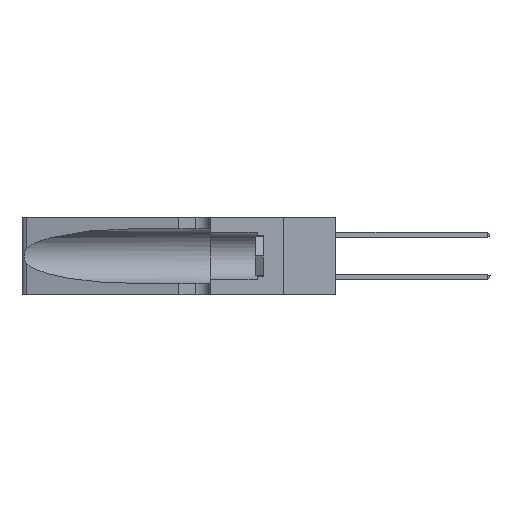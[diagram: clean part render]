
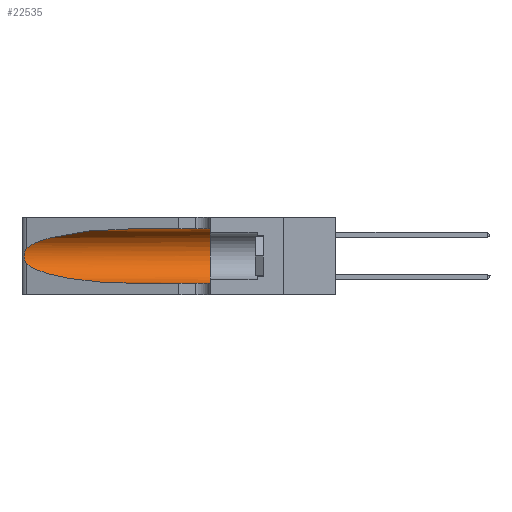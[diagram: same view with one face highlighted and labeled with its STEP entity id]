
A CAD part, left-side view. The second image highlights one B-rep face of the part: STEP entity #22535.
In plain terms, the highlighted cylindrical face has radius 3.308 mm (diameter 6.617 mm), a partial arc.
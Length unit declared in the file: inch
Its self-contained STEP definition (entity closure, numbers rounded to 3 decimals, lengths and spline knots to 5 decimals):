
#37 = ORIENTED_EDGE ( 'NONE', *, *, #28800, .T. ) ;
#1227 = DIRECTION ( 'NONE',  ( 0., 0., 1. ) ) ;
#1616 = CARTESIAN_POINT ( 'NONE',  ( 0.26075, 1.23896, 0.19203 ) ) ;
#3065 = CARTESIAN_POINT ( 'NONE',  ( 0.25487, 1.22718, 0.22369 ) ) ;
#3207 = VECTOR ( 'NONE', #26814, 39.37008 ) ;
#4339 = B_SPLINE_CURVE_WITH_KNOTS ( 'NONE', 3,
 ( #32997, #5074, #39997, #19116, #43518, #22631, #1616, #26113, #5220, #29603, #8793, #33145, #12297, #36642 ),
 .UNSPECIFIED., .F., .F.,
 ( 4, 2, 2, 2, 2, 2, 4 ),
 ( 0., 0.00027, 0.00053, 0.00107, 0.0016, 0.00187, 0.00214 ),
 .UNSPECIFIED. ) ;
#5074 = CARTESIAN_POINT ( 'NONE',  ( 0.25555, 1.22994, 0.2215 ) ) ;
#5168 = LINE ( 'NONE', #7777, #41179 ) ;
#5220 = CARTESIAN_POINT ( 'NONE',  ( 0.26017, 1.23833, 0.17102 ) ) ;
#5455 = LINE ( 'NONE', #9481, #3207 ) ;
#5785 = EDGE_CURVE ( 'NONE', #18991, #15738, #33452, .T. ) ;
#7057 = CARTESIAN_POINT ( 'NONE',  ( 0.18966, 0.96281, 0.05475 ) ) ;
#7777 = CARTESIAN_POINT ( 'NONE',  ( 0.1305, 1.61858, 0.05475 ) ) ;
#8030 = VERTEX_POINT ( 'NONE', #14000 ) ;
#8793 = CARTESIAN_POINT ( 'NONE',  ( 0.25789, 1.23486, 0.15765 ) ) ;
#9481 = CARTESIAN_POINT ( 'NONE',  ( 0.1305, 1.61858, 0.31525 ) ) ;
#12297 = CARTESIAN_POINT ( 'NONE',  ( 0.25555, 1.22993, 0.14849 ) ) ;
#14000 = CARTESIAN_POINT ( 'NONE',  ( 0.25487, 1.22718, 0.14631 ) ) ;
#15154 = AXIS2_PLACEMENT_3D ( 'NONE', #42741, #25344, #28840 ) ;
#15531 = ORIENTED_EDGE ( 'NONE', *, *, #22276, .T. ) ;
#15738 = VERTEX_POINT ( 'NONE', #21286 ) ;
#16546 = VERTEX_POINT ( 'NONE', #43029 ) ;
#17122 = EDGE_CURVE ( 'NONE', #23274, #15738, #5168, .T. ) ;
#18991 = VERTEX_POINT ( 'NONE', #23739 ) ;
#19116 = CARTESIAN_POINT ( 'NONE',  ( 0.25787, 1.23484, 0.2124 ) ) ;
#19890 = ORIENTED_EDGE ( 'NONE', *, *, #17122, .T. ) ;
#21286 = CARTESIAN_POINT ( 'NONE',  ( 0.1305, 0.35, 0.05475 ) ) ;
#21406 = VERTEX_POINT ( 'NONE', #36669 ) ;
#22077 = ORIENTED_EDGE ( 'NONE', *, *, #29671, .F. ) ;
#22264 = DIRECTION ( 'NONE',  ( 0., 1., 0. ) ) ;
#22276 = EDGE_CURVE ( 'NONE', #21406, #16546, #28641, .T. ) ;
#22535 = ADVANCED_FACE ( 'NONE', ( #31312 ), #23187, .F. ) ;
#22631 = CARTESIAN_POINT ( 'NONE',  ( 0.26018, 1.23835, 0.19895 ) ) ;
#23050 = CARTESIAN_POINT ( 'NONE',  ( 0.1305, 0.72297, 0.05475 ) ) ;
#23187 = CYLINDRICAL_SURFACE ( 'NONE', #15154, 0.13025 ) ;
#23274 = VERTEX_POINT ( 'NONE', #23050 ) ;
#23739 = CARTESIAN_POINT ( 'NONE',  ( 0.1305, 0.35, 0.31525 ) ) ;
#24008 = CARTESIAN_POINT ( 'NONE',  ( 0.2373, 1.15595, 0.28018 ) ) ;
#25263 = DIRECTION ( 'NONE',  ( 0., -1., 0. ) ) ;
#25344 = DIRECTION ( 'NONE',  ( 0., -1., 0. ) ) ;
#26113 = CARTESIAN_POINT ( 'NONE',  ( 0.26075, 1.23896, 0.178 ) ) ;
#26814 = DIRECTION ( 'NONE',  ( 0., -1., 0. ) ) ;
#27892 = CARTESIAN_POINT ( 'NONE',  ( 0.2373, 1.15595, 0.08982 ) ) ;
#28026 = ORIENTED_EDGE ( 'NONE', *, *, #33963, .T. ) ;
#28641 =( BOUNDED_CURVE ( )  B_SPLINE_CURVE ( 3, ( #37874, #41381, #24008, #3065 ),
 .UNSPECIFIED., .F., .F. ) 
 B_SPLINE_CURVE_WITH_KNOTS ( ( 4, 4 ),
 ( 1.5708, 2.84003 ),
 .UNSPECIFIED. ) 
 CURVE ( )  GEOMETRIC_REPRESENTATION_ITEM ( )  RATIONAL_B_SPLINE_CURVE ( ( 1., 0.87, 0.87, 1. ) ) 
 REPRESENTATION_ITEM ( '' )  );
#28800 = EDGE_CURVE ( 'NONE', #16546, #8030, #4339, .T. ) ;
#28840 = DIRECTION ( 'NONE',  ( 0., 0., -1. ) ) ;
#29603 = CARTESIAN_POINT ( 'NONE',  ( 0.25856, 1.23593, 0.16098 ) ) ;
#29671 = EDGE_CURVE ( 'NONE', #21406, #18991, #5455, .T. ) ;
#31312 = FACE_OUTER_BOUND ( 'NONE', #42839, .T. ) ;
#31399 = CARTESIAN_POINT ( 'NONE',  ( 0.1305, 0.72297, 0.05475 ) ) ;
#32997 = CARTESIAN_POINT ( 'NONE',  ( 0.25487, 1.22718, 0.22369 ) ) ;
#33145 = CARTESIAN_POINT ( 'NONE',  ( 0.25639, 1.23186, 0.15144 ) ) ;
#33446 =( BOUNDED_CURVE ( )  B_SPLINE_CURVE ( 3, ( #45306, #27892, #7057, #31399 ),
 .UNSPECIFIED., .F., .F. ) 
 B_SPLINE_CURVE_WITH_KNOTS ( ( 4, 4 ),
 ( 3.44316, 4.71239 ),
 .UNSPECIFIED. ) 
 CURVE ( )  GEOMETRIC_REPRESENTATION_ITEM ( )  RATIONAL_B_SPLINE_CURVE ( ( 1., 0.87, 0.87, 1. ) ) 
 REPRESENTATION_ITEM ( '' )  );
#33452 = CIRCLE ( 'NONE', #40711, 0.13025 ) ;
#33963 = EDGE_CURVE ( 'NONE', #8030, #23274, #33446, .T. ) ;
#36642 = CARTESIAN_POINT ( 'NONE',  ( 0.25487, 1.22718, 0.14631 ) ) ;
#36669 = CARTESIAN_POINT ( 'NONE',  ( 0.1305, 0.72297, 0.31525 ) ) ;
#37874 = CARTESIAN_POINT ( 'NONE',  ( 0.1305, 0.72297, 0.31525 ) ) ;
#39520 = ORIENTED_EDGE ( 'NONE', *, *, #5785, .F. ) ;
#39997 = CARTESIAN_POINT ( 'NONE',  ( 0.25639, 1.23184, 0.21858 ) ) ;
#40711 = AXIS2_PLACEMENT_3D ( 'NONE', #43157, #22264, #1227 ) ;
#41179 = VECTOR ( 'NONE', #25263, 39.37008 ) ;
#41381 = CARTESIAN_POINT ( 'NONE',  ( 0.18966, 0.96281, 0.31525 ) ) ;
#42741 = CARTESIAN_POINT ( 'NONE',  ( 0.1305, 1.61858, 0.185 ) ) ;
#42839 = EDGE_LOOP ( 'NONE', ( #15531, #37, #28026, #19890, #39520, #22077 ) ) ;
#43029 = CARTESIAN_POINT ( 'NONE',  ( 0.25487, 1.22718, 0.22369 ) ) ;
#43157 = CARTESIAN_POINT ( 'NONE',  ( 0.1305, 0.35, 0.185 ) ) ;
#43518 = CARTESIAN_POINT ( 'NONE',  ( 0.25854, 1.2359, 0.20912 ) ) ;
#45306 = CARTESIAN_POINT ( 'NONE',  ( 0.25487, 1.22718, 0.14631 ) ) ;
